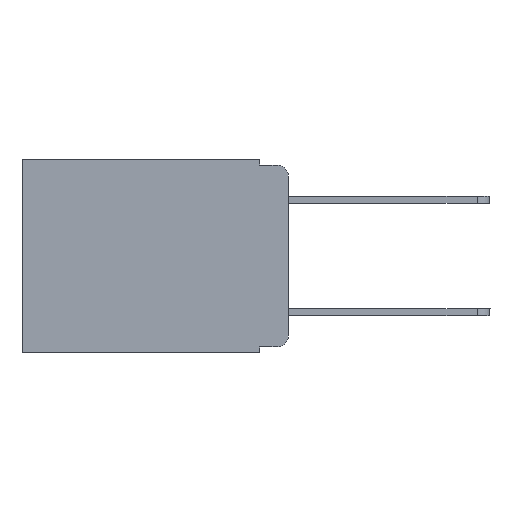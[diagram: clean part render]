
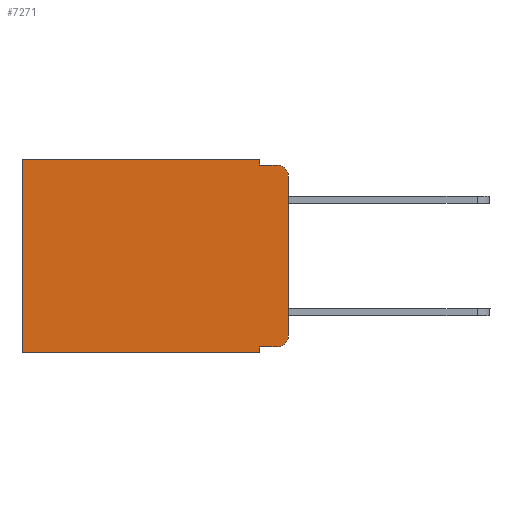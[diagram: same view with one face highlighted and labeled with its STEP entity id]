
A CAD part, left-side view. The second image highlights one B-rep face of the part: STEP entity #7271.
In plain terms, the highlighted planar face has unit normal (-1, 0, 0).
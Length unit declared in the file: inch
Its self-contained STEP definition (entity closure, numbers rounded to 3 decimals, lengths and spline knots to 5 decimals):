
#208 = CARTESIAN_POINT ( 'NONE',  ( 0.298, 0.02, -0.01 ) ) ;
#429 = DIRECTION ( 'NONE',  ( 0., 0., -1. ) ) ;
#538 = ORIENTED_EDGE ( 'NONE', *, *, #21246, .T. ) ;
#983 = VECTOR ( 'NONE', #429, 39.37008 ) ;
#1346 = ORIENTED_EDGE ( 'NONE', *, *, #6908, .T. ) ;
#1560 = VERTEX_POINT ( 'NONE', #5784 ) ;
#1719 = CARTESIAN_POINT ( 'NONE',  ( 0.298, 0.02, -0.313 ) ) ;
#2220 = DIRECTION ( 'NONE',  ( -1., 0., 0. ) ) ;
#2301 = LINE ( 'NONE', #11307, #4501 ) ;
#2496 = ORIENTED_EDGE ( 'NONE', *, *, #19672, .T. ) ;
#2856 = ORIENTED_EDGE ( 'NONE', *, *, #12242, .F. ) ;
#2858 = DIRECTION ( 'NONE',  ( 0., 0., -1. ) ) ;
#3887 = VECTOR ( 'NONE', #7683, 39.37008 ) ;
#4225 = DIRECTION ( 'NONE',  ( 0., 0., -1. ) ) ;
#4501 = VECTOR ( 'NONE', #13582, 39.37008 ) ;
#5122 = LINE ( 'NONE', #8688, #25495 ) ;
#5664 = VERTEX_POINT ( 'NONE', #20893 ) ;
#5784 = CARTESIAN_POINT ( 'NONE',  ( 0.298, 0.473, 0. ) ) ;
#5973 = CARTESIAN_POINT ( 'NONE',  ( 0.298, 0., -0.313 ) ) ;
#6036 = LINE ( 'NONE', #15308, #3887 ) ;
#6326 = CARTESIAN_POINT ( 'NONE',  ( 0.298, 0., -0.343 ) ) ;
#6462 = VECTOR ( 'NONE', #17970, 39.37008 ) ;
#6573 = ORIENTED_EDGE ( 'NONE', *, *, #17588, .F. ) ;
#6862 = VERTEX_POINT ( 'NONE', #16146 ) ;
#6908 = EDGE_CURVE ( 'NONE', #10568, #18722, #12209, .T. ) ;
#7050 = CARTESIAN_POINT ( 'NONE',  ( 0.298, 0., 0. ) ) ;
#7141 = EDGE_CURVE ( 'NONE', #22384, #5664, #5122, .T. ) ;
#7271 = ADVANCED_FACE ( 'NONE', ( #9427 ), #11442, .F. ) ;
#7465 = CARTESIAN_POINT ( 'NONE',  ( 0.298, 0.051, -0.333 ) ) ;
#7467 = CARTESIAN_POINT ( 'NONE',  ( 0.298, 0., -0.03 ) ) ;
#7683 = DIRECTION ( 'NONE',  ( 0., -1., 0. ) ) ;
#7738 = ORIENTED_EDGE ( 'NONE', *, *, #7141, .T. ) ;
#8298 = ORIENTED_EDGE ( 'NONE', *, *, #10749, .F. ) ;
#8688 = CARTESIAN_POINT ( 'NONE',  ( 0.298, 0.051, -0.333 ) ) ;
#8751 = VECTOR ( 'NONE', #2858, 39.37008 ) ;
#9279 = CARTESIAN_POINT ( 'NONE',  ( 0.298, 0.473, 0. ) ) ;
#9375 = EDGE_LOOP ( 'NONE', ( #8298, #1346, #17074, #6573, #538, #16588, #2856, #9723, #7738, #2496 ) ) ;
#9427 = FACE_OUTER_BOUND ( 'NONE', #9375, .T. ) ;
#9723 = ORIENTED_EDGE ( 'NONE', *, *, #22893, .F. ) ;
#9726 = DIRECTION ( 'NONE',  ( 0., 0., -1. ) ) ;
#10568 = VERTEX_POINT ( 'NONE', #7467 ) ;
#10749 = EDGE_CURVE ( 'NONE', #10568, #14707, #22578, .T. ) ;
#10792 = LINE ( 'NONE', #6326, #6462 ) ;
#10968 = CARTESIAN_POINT ( 'NONE',  ( 0.298, 0.051, 0. ) ) ;
#11307 = CARTESIAN_POINT ( 'NONE',  ( 0.298, 0., 0. ) ) ;
#11442 = PLANE ( 'NONE',  #25153 ) ;
#11529 = LINE ( 'NONE', #10968, #8751 ) ;
#12209 = CIRCLE ( 'NONE', #18686, 0.02 ) ;
#12242 = EDGE_CURVE ( 'NONE', #6862, #19003, #10792, .T. ) ;
#13434 = CARTESIAN_POINT ( 'NONE',  ( 0.298, 0.473, -0.343 ) ) ;
#13582 = DIRECTION ( 'NONE',  ( 0., 1., 0. ) ) ;
#13778 = LINE ( 'NONE', #9279, #21464 ) ;
#14081 = CARTESIAN_POINT ( 'NONE',  ( 0.298, 0.02, -0.03 ) ) ;
#14616 = CARTESIAN_POINT ( 'NONE',  ( 0.298, 0.051, 0. ) ) ;
#14707 = VERTEX_POINT ( 'NONE', #5973 ) ;
#15161 = AXIS2_PLACEMENT_3D ( 'NONE', #1719, #25190, #9726 ) ;
#15272 = DIRECTION ( 'NONE',  ( 0., 0., -1. ) ) ;
#15308 = CARTESIAN_POINT ( 'NONE',  ( 0.298, 0.051, -0.01 ) ) ;
#15769 = EDGE_CURVE ( 'NONE', #1560, #19003, #13778, .T. ) ;
#16146 = CARTESIAN_POINT ( 'NONE',  ( 0.298, 0.051, -0.343 ) ) ;
#16364 = CIRCLE ( 'NONE', #15161, 0.02 ) ;
#16588 = ORIENTED_EDGE ( 'NONE', *, *, #15769, .T. ) ;
#16736 = DIRECTION ( 'NONE',  ( 0., -1., 0. ) ) ;
#17074 = ORIENTED_EDGE ( 'NONE', *, *, #21287, .F. ) ;
#17588 = EDGE_CURVE ( 'NONE', #20290, #19589, #22282, .T. ) ;
#17970 = DIRECTION ( 'NONE',  ( 0., 1., 0. ) ) ;
#18261 = VECTOR ( 'NONE', #24898, 39.37008 ) ;
#18686 = AXIS2_PLACEMENT_3D ( 'NONE', #14081, #2220, #4225 ) ;
#18722 = VERTEX_POINT ( 'NONE', #208 ) ;
#19003 = VERTEX_POINT ( 'NONE', #13434 ) ;
#19044 = CARTESIAN_POINT ( 'NONE',  ( 0.298, 0.051, 0. ) ) ;
#19589 = VERTEX_POINT ( 'NONE', #24939 ) ;
#19672 = EDGE_CURVE ( 'NONE', #5664, #14707, #16364, .T. ) ;
#20290 = VERTEX_POINT ( 'NONE', #19044 ) ;
#20893 = CARTESIAN_POINT ( 'NONE',  ( 0.298, 0.02, -0.333 ) ) ;
#21246 = EDGE_CURVE ( 'NONE', #20290, #1560, #2301, .T. ) ;
#21287 = EDGE_CURVE ( 'NONE', #19589, #18722, #6036, .T. ) ;
#21464 = VECTOR ( 'NONE', #23328, 39.37008 ) ;
#22282 = LINE ( 'NONE', #14616, #983 ) ;
#22384 = VERTEX_POINT ( 'NONE', #7465 ) ;
#22578 = LINE ( 'NONE', #7050, #18261 ) ;
#22893 = EDGE_CURVE ( 'NONE', #22384, #6862, #11529, .T. ) ;
#22905 = CARTESIAN_POINT ( 'NONE',  ( 0.298, 0., 0. ) ) ;
#23328 = DIRECTION ( 'NONE',  ( 0., 0., -1. ) ) ;
#24898 = DIRECTION ( 'NONE',  ( 0., 0., -1. ) ) ;
#24910 = DIRECTION ( 'NONE',  ( 1., 0., 0. ) ) ;
#24939 = CARTESIAN_POINT ( 'NONE',  ( 0.298, 0.051, -0.01 ) ) ;
#25153 = AXIS2_PLACEMENT_3D ( 'NONE', #22905, #24910, #15272 ) ;
#25190 = DIRECTION ( 'NONE',  ( -1., 0., 0. ) ) ;
#25495 = VECTOR ( 'NONE', #16736, 39.37008 ) ;
